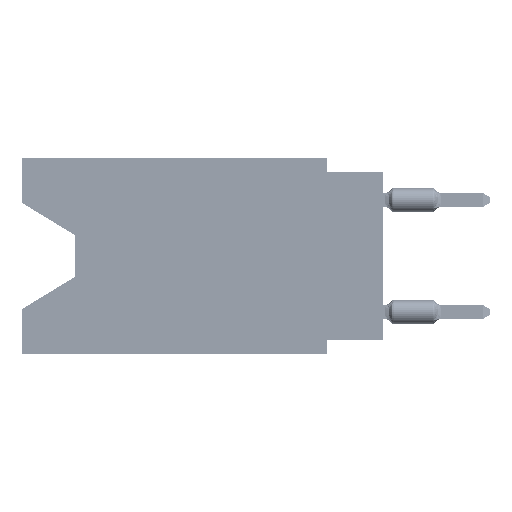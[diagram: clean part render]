
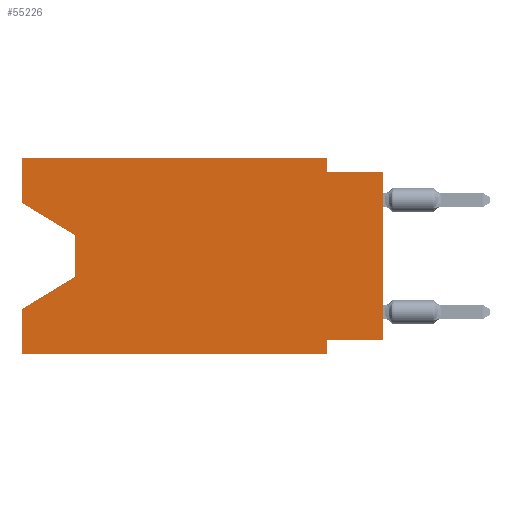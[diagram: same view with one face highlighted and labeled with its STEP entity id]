
A CAD part, left-side view. The second image highlights one B-rep face of the part: STEP entity #55226.
In plain terms, the highlighted planar face has unit normal (-1, 0, 0).
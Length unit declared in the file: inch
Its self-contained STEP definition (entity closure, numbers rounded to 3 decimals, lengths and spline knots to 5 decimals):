
#1833 = CARTESIAN_POINT ( 'NONE',  ( 0., 0.1, -0.325 ) ) ;
#2940 = CARTESIAN_POINT ( 'NONE',  ( 0., 0.55, -0.212 ) ) ;
#3644 = VECTOR ( 'NONE', #45669, 39.37008 ) ;
#4189 = VERTEX_POINT ( 'NONE', #58285 ) ;
#4804 = VERTEX_POINT ( 'NONE', #57475 ) ;
#4817 = CARTESIAN_POINT ( 'NONE',  ( 0., 0.1, -0.025 ) ) ;
#5435 = EDGE_CURVE ( 'NONE', #67082, #31914, #47415, .T. ) ;
#6350 = DIRECTION ( 'NONE',  ( 0., 0., -1. ) ) ;
#7444 = VERTEX_POINT ( 'NONE', #2940 ) ;
#8118 = VECTOR ( 'NONE', #64224, 39.37008 ) ;
#8805 = EDGE_CURVE ( 'NONE', #55609, #56776, #28025, .T. ) ;
#8987 = LINE ( 'NONE', #60350, #13849 ) ;
#9738 = LINE ( 'NONE', #65568, #3644 ) ;
#9839 = VERTEX_POINT ( 'NONE', #50104 ) ;
#9945 = LINE ( 'NONE', #41399, #41075 ) ;
#10370 = CARTESIAN_POINT ( 'NONE',  ( 0., 0.645, 0. ) ) ;
#10832 = VERTEX_POINT ( 'NONE', #20701 ) ;
#10834 = CARTESIAN_POINT ( 'NONE',  ( 0., 0.645, 0. ) ) ;
#12002 = CARTESIAN_POINT ( 'NONE',  ( 0., 0.645, -0.35 ) ) ;
#12434 = VECTOR ( 'NONE', #55883, 39.37008 ) ;
#13849 = VECTOR ( 'NONE', #50752, 39.37008 ) ;
#14786 = CARTESIAN_POINT ( 'NONE',  ( 0., 0., 0. ) ) ;
#15972 = LINE ( 'NONE', #26250, #8118 ) ;
#16359 = EDGE_CURVE ( 'NONE', #7444, #31914, #9945, .T. ) ;
#17063 = CARTESIAN_POINT ( 'NONE',  ( 0., 0.1, -0.35 ) ) ;
#17926 = CARTESIAN_POINT ( 'NONE',  ( 0., 0.1, -0.35 ) ) ;
#20575 = CARTESIAN_POINT ( 'NONE',  ( 0., 0., -0.025 ) ) ;
#20701 = CARTESIAN_POINT ( 'NONE',  ( 0., 0., -0.025 ) ) ;
#21164 = CARTESIAN_POINT ( 'NONE',  ( 0., 0.645, -0.08025 ) ) ;
#21599 = DIRECTION ( 'NONE',  ( 0., -1., 0. ) ) ;
#21754 = CARTESIAN_POINT ( 'NONE',  ( 0., 0.645, -0.26975 ) ) ;
#22381 = EDGE_CURVE ( 'NONE', #23511, #41006, #15972, .T. ) ;
#22407 = ORIENTED_EDGE ( 'NONE', *, *, #48060, .T. ) ;
#23511 = VERTEX_POINT ( 'NONE', #61627 ) ;
#25746 = ORIENTED_EDGE ( 'NONE', *, *, #28194, .T. ) ;
#26250 = CARTESIAN_POINT ( 'NONE',  ( 0., 0.645, 0. ) ) ;
#27342 = DIRECTION ( 'NONE',  ( 0., 0., -1. ) ) ;
#27697 = EDGE_CURVE ( 'NONE', #23511, #9839, #41699, .T. ) ;
#28025 = LINE ( 'NONE', #17063, #58589 ) ;
#28194 = EDGE_CURVE ( 'NONE', #67082, #56776, #42452, .T. ) ;
#28286 = CARTESIAN_POINT ( 'NONE',  ( 0., 0.645, 0. ) ) ;
#29841 = LINE ( 'NONE', #50732, #12434 ) ;
#30595 = ORIENTED_EDGE ( 'NONE', *, *, #38836, .F. ) ;
#31267 = ORIENTED_EDGE ( 'NONE', *, *, #27697, .T. ) ;
#31914 = VERTEX_POINT ( 'NONE', #21754 ) ;
#32573 = CARTESIAN_POINT ( 'NONE',  ( 0., 0.645, -0.35 ) ) ;
#32714 = VECTOR ( 'NONE', #52747, 39.37008 ) ;
#34338 = DIRECTION ( 'NONE',  ( 0., 0., -1. ) ) ;
#34573 = ORIENTED_EDGE ( 'NONE', *, *, #5435, .F. ) ;
#35467 = EDGE_CURVE ( 'NONE', #52897, #10832, #63354, .T. ) ;
#36531 = ORIENTED_EDGE ( 'NONE', *, *, #35467, .F. ) ;
#36930 = VECTOR ( 'NONE', #34338, 39.37008 ) ;
#37813 = AXIS2_PLACEMENT_3D ( 'NONE', #28286, #44325, #6350 ) ;
#38836 = EDGE_CURVE ( 'NONE', #4189, #52897, #48161, .T. ) ;
#40301 = ORIENTED_EDGE ( 'NONE', *, *, #45406, .T. ) ;
#41006 = VERTEX_POINT ( 'NONE', #10370 ) ;
#41075 = VECTOR ( 'NONE', #51050, 39.37008 ) ;
#41399 = CARTESIAN_POINT ( 'NONE',  ( 0., 0.55, -0.212 ) ) ;
#41699 = LINE ( 'NONE', #21164, #54495 ) ;
#42452 = LINE ( 'NONE', #12002, #61086 ) ;
#43671 = ORIENTED_EDGE ( 'NONE', *, *, #22381, .F. ) ;
#44325 = DIRECTION ( 'NONE',  ( 1., 0., 0. ) ) ;
#45299 = CARTESIAN_POINT ( 'NONE',  ( 0., 0.1, 0. ) ) ;
#45406 = EDGE_CURVE ( 'NONE', #4804, #10832, #52094, .T. ) ;
#45669 = DIRECTION ( 'NONE',  ( 0., 0., -1. ) ) ;
#47415 = LINE ( 'NONE', #10834, #53887 ) ;
#47685 = VECTOR ( 'NONE', #57880, 39.37008 ) ;
#48060 = EDGE_CURVE ( 'NONE', #9839, #7444, #9738, .T. ) ;
#48161 = LINE ( 'NONE', #45299, #36930 ) ;
#48475 = EDGE_CURVE ( 'NONE', #4804, #55609, #29841, .T. ) ;
#50104 = CARTESIAN_POINT ( 'NONE',  ( 0., 0.55, -0.138 ) ) ;
#50732 = CARTESIAN_POINT ( 'NONE',  ( 0., 0., -0.325 ) ) ;
#50752 = DIRECTION ( 'NONE',  ( 0., -1., 0. ) ) ;
#51050 = DIRECTION ( 'NONE',  ( 0., 0.855, -0.519 ) ) ;
#52094 = LINE ( 'NONE', #14786, #32714 ) ;
#52747 = DIRECTION ( 'NONE',  ( 0., 0., 1. ) ) ;
#52897 = VERTEX_POINT ( 'NONE', #4817 ) ;
#53274 = PLANE ( 'NONE',  #37813 ) ;
#53887 = VECTOR ( 'NONE', #58061, 39.37008 ) ;
#53926 = FACE_OUTER_BOUND ( 'NONE', #54330, .T. ) ;
#54330 = EDGE_LOOP ( 'NONE', ( #31267, #22407, #62618, #34573, #25746, #60375, #58814, #40301, #36531, #30595, #60807, #43671 ) ) ;
#54495 = VECTOR ( 'NONE', #62302, 39.37008 ) ;
#55226 = ADVANCED_FACE ( 'NONE', ( #53926 ), #53274, .F. ) ;
#55609 = VERTEX_POINT ( 'NONE', #1833 ) ;
#55716 = EDGE_CURVE ( 'NONE', #41006, #4189, #8987, .T. ) ;
#55883 = DIRECTION ( 'NONE',  ( 0., 1., 0. ) ) ;
#56776 = VERTEX_POINT ( 'NONE', #17926 ) ;
#57475 = CARTESIAN_POINT ( 'NONE',  ( 0., 0., -0.325 ) ) ;
#57880 = DIRECTION ( 'NONE',  ( 0., -1., 0. ) ) ;
#58061 = DIRECTION ( 'NONE',  ( 0., 0., 1. ) ) ;
#58285 = CARTESIAN_POINT ( 'NONE',  ( 0., 0.1, 0. ) ) ;
#58589 = VECTOR ( 'NONE', #27342, 39.37008 ) ;
#58814 = ORIENTED_EDGE ( 'NONE', *, *, #48475, .F. ) ;
#60350 = CARTESIAN_POINT ( 'NONE',  ( 0., 0.645, 0. ) ) ;
#60375 = ORIENTED_EDGE ( 'NONE', *, *, #8805, .F. ) ;
#60807 = ORIENTED_EDGE ( 'NONE', *, *, #55716, .F. ) ;
#61086 = VECTOR ( 'NONE', #21599, 39.37008 ) ;
#61627 = CARTESIAN_POINT ( 'NONE',  ( 0., 0.645, -0.08025 ) ) ;
#62302 = DIRECTION ( 'NONE',  ( 0., -0.855, -0.519 ) ) ;
#62618 = ORIENTED_EDGE ( 'NONE', *, *, #16359, .T. ) ;
#63354 = LINE ( 'NONE', #20575, #47685 ) ;
#64224 = DIRECTION ( 'NONE',  ( 0., 0., 1. ) ) ;
#65568 = CARTESIAN_POINT ( 'NONE',  ( 0., 0.55, -0.138 ) ) ;
#67082 = VERTEX_POINT ( 'NONE', #32573 ) ;
